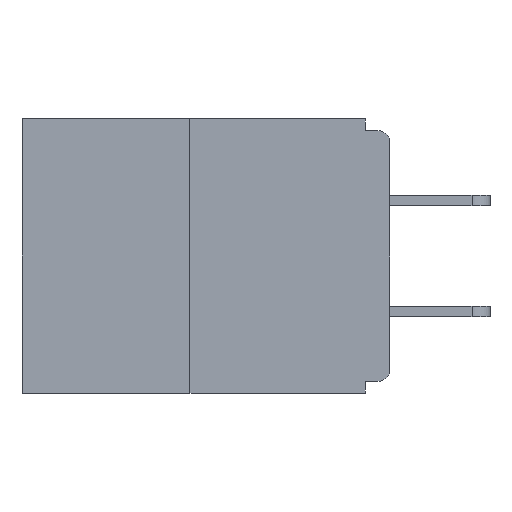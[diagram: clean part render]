
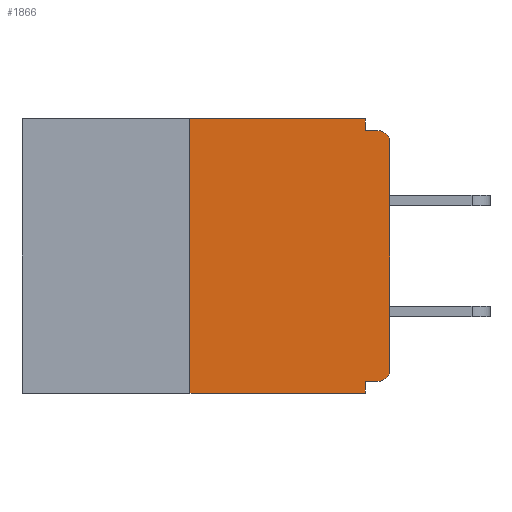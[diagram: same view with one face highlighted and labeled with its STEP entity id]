
A CAD part, left-side view. The second image highlights one B-rep face of the part: STEP entity #1866.
In plain terms, the highlighted planar face has unit normal (-1, 0, 0).
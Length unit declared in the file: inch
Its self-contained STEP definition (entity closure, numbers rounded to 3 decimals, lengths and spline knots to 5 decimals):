
#235 = VECTOR ( 'NONE', #15766, 39.37008 ) ;
#244 = AXIS2_PLACEMENT_3D ( 'NONE', #18137, #26031, #13906 ) ;
#245 = DIRECTION ( 'NONE',  ( 0., -1., 0. ) ) ;
#265 = LINE ( 'NONE', #6653, #25154 ) ;
#584 = VERTEX_POINT ( 'NONE', #21130 ) ;
#1060 = ORIENTED_EDGE ( 'NONE', *, *, #18807, .F. ) ;
#1851 = AXIS2_PLACEMENT_3D ( 'NONE', #10197, #26023, #24339 ) ;
#1866 = ADVANCED_FACE ( 'NONE', ( #16325 ), #4052, .F. ) ;
#1931 = LINE ( 'NONE', #17148, #5091 ) ;
#2098 = VERTEX_POINT ( 'NONE', #19526 ) ;
#2628 = AXIS2_PLACEMENT_3D ( 'NONE', #16918, #12618, #16668 ) ;
#2659 = LINE ( 'NONE', #24105, #9875 ) ;
#2689 = DIRECTION ( 'NONE',  ( 0., 0., 1. ) ) ;
#3328 = ORIENTED_EDGE ( 'NONE', *, *, #24751, .T. ) ;
#4051 = LINE ( 'NONE', #19575, #235 ) ;
#4052 = PLANE ( 'NONE',  #244 ) ;
#4134 = ORIENTED_EDGE ( 'NONE', *, *, #4977, .T. ) ;
#4573 = VERTEX_POINT ( 'NONE', #25318 ) ;
#4977 = EDGE_CURVE ( 'NONE', #17903, #6365, #12996, .T. ) ;
#5049 = ORIENTED_EDGE ( 'NONE', *, *, #18221, .T. ) ;
#5091 = VECTOR ( 'NONE', #23439, 39.37008 ) ;
#5154 = LINE ( 'NONE', #5937, #25989 ) ;
#5472 = CIRCLE ( 'NONE', #2628, 0.015 ) ;
#5646 = ORIENTED_EDGE ( 'NONE', *, *, #21641, .F. ) ;
#5937 = CARTESIAN_POINT ( 'NONE',  ( 0., 0., -0.015 ) ) ;
#6101 = EDGE_CURVE ( 'NONE', #7136, #15245, #13859, .T. ) ;
#6365 = VERTEX_POINT ( 'NONE', #23783 ) ;
#6653 = CARTESIAN_POINT ( 'NONE',  ( 0., 0.25, 0. ) ) ;
#7136 = VERTEX_POINT ( 'NONE', #24025 ) ;
#7577 = VERTEX_POINT ( 'NONE', #16905 ) ;
#9407 = VERTEX_POINT ( 'NONE', #9837 ) ;
#9837 = CARTESIAN_POINT ( 'NONE',  ( 0., 0.25, -0.343 ) ) ;
#9875 = VECTOR ( 'NONE', #13997, 39.37008 ) ;
#10084 = ORIENTED_EDGE ( 'NONE', *, *, #6101, .F. ) ;
#10197 = CARTESIAN_POINT ( 'NONE',  ( 0., 0.015, -0.313 ) ) ;
#10624 = EDGE_CURVE ( 'NONE', #15245, #25613, #1931, .T. ) ;
#11636 = VECTOR ( 'NONE', #16857, 39.37008 ) ;
#11910 = CIRCLE ( 'NONE', #1851, 0.015 ) ;
#12618 = DIRECTION ( 'NONE',  ( -1., 0., 0. ) ) ;
#12996 = LINE ( 'NONE', #14553, #24389 ) ;
#13859 = LINE ( 'NONE', #18168, #21795 ) ;
#13906 = DIRECTION ( 'NONE',  ( 0., 0., -1. ) ) ;
#13997 = DIRECTION ( 'NONE',  ( 0., -1., 0. ) ) ;
#14454 = DIRECTION ( 'NONE',  ( 0., 1., 0. ) ) ;
#14553 = CARTESIAN_POINT ( 'NONE',  ( 0., 0., 0. ) ) ;
#14586 = CARTESIAN_POINT ( 'NONE',  ( 0., 0.031, -0.328 ) ) ;
#15245 = VERTEX_POINT ( 'NONE', #14586 ) ;
#15250 = CARTESIAN_POINT ( 'NONE',  ( 0., 0.031, -0.343 ) ) ;
#15766 = DIRECTION ( 'NONE',  ( 0., -1., 0. ) ) ;
#16325 = FACE_OUTER_BOUND ( 'NONE', #19308, .T. ) ;
#16668 = DIRECTION ( 'NONE',  ( 0., 0., -1. ) ) ;
#16857 = DIRECTION ( 'NONE',  ( 0., 0., -1. ) ) ;
#16905 = CARTESIAN_POINT ( 'NONE',  ( 0., 0.015, -0.015 ) ) ;
#16918 = CARTESIAN_POINT ( 'NONE',  ( 0., 0.015, -0.03 ) ) ;
#17040 = EDGE_CURVE ( 'NONE', #584, #2098, #25853, .T. ) ;
#17148 = CARTESIAN_POINT ( 'NONE',  ( 0., 0.031, -0.343 ) ) ;
#17903 = VERTEX_POINT ( 'NONE', #25397 ) ;
#18137 = CARTESIAN_POINT ( 'NONE',  ( 0., 0.46, 0. ) ) ;
#18168 = CARTESIAN_POINT ( 'NONE',  ( 0., 0., -0.328 ) ) ;
#18221 = EDGE_CURVE ( 'NONE', #7136, #17903, #11910, .T. ) ;
#18807 = EDGE_CURVE ( 'NONE', #2098, #7577, #5154, .T. ) ;
#19308 = EDGE_LOOP ( 'NONE', ( #22212, #5646, #19505, #22050, #10084, #5049, #4134, #3328, #1060, #24557 ) ) ;
#19505 = ORIENTED_EDGE ( 'NONE', *, *, #24593, .T. ) ;
#19526 = CARTESIAN_POINT ( 'NONE',  ( 0., 0.031, -0.015 ) ) ;
#19575 = CARTESIAN_POINT ( 'NONE',  ( 0., 0.46, 0. ) ) ;
#21130 = CARTESIAN_POINT ( 'NONE',  ( 0., 0.031, 0. ) ) ;
#21641 = EDGE_CURVE ( 'NONE', #9407, #4573, #265, .T. ) ;
#21795 = VECTOR ( 'NONE', #14454, 39.37008 ) ;
#22050 = ORIENTED_EDGE ( 'NONE', *, *, #10624, .F. ) ;
#22212 = ORIENTED_EDGE ( 'NONE', *, *, #24978, .F. ) ;
#22366 = CARTESIAN_POINT ( 'NONE',  ( 0., 0.031, 0. ) ) ;
#23439 = DIRECTION ( 'NONE',  ( 0., 0., -1. ) ) ;
#23783 = CARTESIAN_POINT ( 'NONE',  ( 0., 0., -0.03 ) ) ;
#24025 = CARTESIAN_POINT ( 'NONE',  ( 0., 0.015, -0.328 ) ) ;
#24105 = CARTESIAN_POINT ( 'NONE',  ( 0., 0.46, -0.343 ) ) ;
#24339 = DIRECTION ( 'NONE',  ( 0., 0., -1. ) ) ;
#24389 = VECTOR ( 'NONE', #24743, 39.37008 ) ;
#24557 = ORIENTED_EDGE ( 'NONE', *, *, #17040, .F. ) ;
#24593 = EDGE_CURVE ( 'NONE', #9407, #25613, #2659, .T. ) ;
#24743 = DIRECTION ( 'NONE',  ( 0., 0., 1. ) ) ;
#24751 = EDGE_CURVE ( 'NONE', #6365, #7577, #5472, .T. ) ;
#24978 = EDGE_CURVE ( 'NONE', #4573, #584, #4051, .T. ) ;
#25154 = VECTOR ( 'NONE', #2689, 39.37008 ) ;
#25318 = CARTESIAN_POINT ( 'NONE',  ( 0., 0.25, 0. ) ) ;
#25397 = CARTESIAN_POINT ( 'NONE',  ( 0., 0., -0.313 ) ) ;
#25613 = VERTEX_POINT ( 'NONE', #15250 ) ;
#25853 = LINE ( 'NONE', #22366, #11636 ) ;
#25989 = VECTOR ( 'NONE', #245, 39.37008 ) ;
#26023 = DIRECTION ( 'NONE',  ( -1., 0., 0. ) ) ;
#26031 = DIRECTION ( 'NONE',  ( 1., 0., 0. ) ) ;
